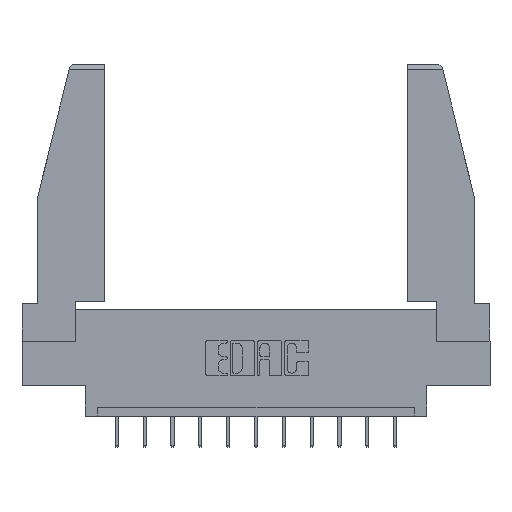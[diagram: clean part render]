
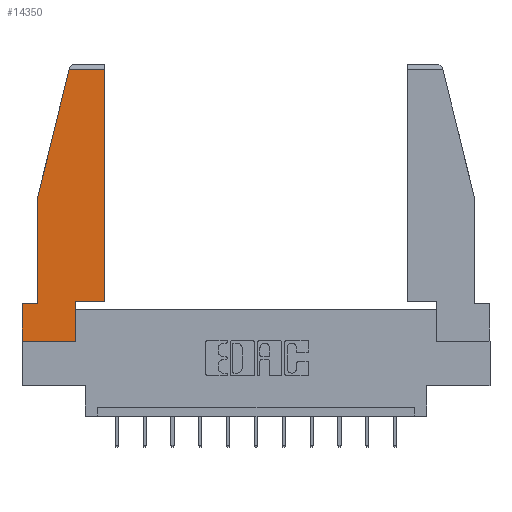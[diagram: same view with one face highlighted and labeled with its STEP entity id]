
A CAD part, top view. The second image highlights one B-rep face of the part: STEP entity #14350.
In plain terms, the highlighted planar face has unit normal (0, 0, 1).
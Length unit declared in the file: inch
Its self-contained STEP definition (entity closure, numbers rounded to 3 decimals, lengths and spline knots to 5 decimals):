
#652 = EDGE_CURVE ( 'NONE', #4869, #4656, #8339, .T. ) ;
#977 = EDGE_CURVE ( 'NONE', #4656, #2754, #12993, .T. ) ;
#1386 = DIRECTION ( 'NONE',  ( 1., 0., 0. ) ) ;
#1557 = ORIENTED_EDGE ( 'NONE', *, *, #977, .T. ) ;
#1839 = VECTOR ( 'NONE', #2332, 39.37008 ) ;
#2135 = FACE_OUTER_BOUND ( 'NONE', #13114, .T. ) ;
#2332 = DIRECTION ( 'NONE',  ( 0., 1., 0. ) ) ;
#2437 = DIRECTION ( 'NONE',  ( -1., 0., 0. ) ) ;
#2501 = DIRECTION ( 'NONE',  ( 0., 1., 0. ) ) ;
#2518 = VERTEX_POINT ( 'NONE', #7886 ) ;
#2739 = ORIENTED_EDGE ( 'NONE', *, *, #652, .T. ) ;
#2754 = VERTEX_POINT ( 'NONE', #12112 ) ;
#3311 = CARTESIAN_POINT ( 'NONE',  ( 0., 0., 0. ) ) ;
#3461 = LINE ( 'NONE', #5971, #7986 ) ;
#3486 = CARTESIAN_POINT ( 'NONE',  ( 0.461, 1.52, 0. ) ) ;
#3615 = DIRECTION ( 'NONE',  ( 0., 0., 1. ) ) ;
#3895 = ORIENTED_EDGE ( 'NONE', *, *, #5594, .T. ) ;
#4079 = ORIENTED_EDGE ( 'NONE', *, *, #12939, .T. ) ;
#4114 = CARTESIAN_POINT ( 'NONE',  ( 0.086, 0.21, 0. ) ) ;
#4650 = VECTOR ( 'NONE', #9243, 39.37008 ) ;
#4656 = VERTEX_POINT ( 'NONE', #4114 ) ;
#4683 = DIRECTION ( 'NONE',  ( 0., -1., 0. ) ) ;
#4845 = VERTEX_POINT ( 'NONE', #10705 ) ;
#4869 = VERTEX_POINT ( 'NONE', #10540 ) ;
#4885 = LINE ( 'NONE', #13971, #1839 ) ;
#4939 = PLANE ( 'NONE',  #11507 ) ;
#5016 = LINE ( 'NONE', #14235, #9665 ) ;
#5052 = CARTESIAN_POINT ( 'NONE',  ( 0.2636, 1.52, 0. ) ) ;
#5412 = ORIENTED_EDGE ( 'NONE', *, *, #7870, .T. ) ;
#5594 = EDGE_CURVE ( 'NONE', #6799, #10793, #7722, .T. ) ;
#5870 = CARTESIAN_POINT ( 'NONE',  ( 0., 0.21, 0. ) ) ;
#5971 = CARTESIAN_POINT ( 'NONE',  ( 0.461, 0.223, 0. ) ) ;
#6303 = ORIENTED_EDGE ( 'NONE', *, *, #13907, .T. ) ;
#6676 = ORIENTED_EDGE ( 'NONE', *, *, #7749, .T. ) ;
#6799 = VERTEX_POINT ( 'NONE', #3311 ) ;
#7091 = CARTESIAN_POINT ( 'NONE',  ( 0., 0., 0. ) ) ;
#7204 = VERTEX_POINT ( 'NONE', #3486 ) ;
#7722 = LINE ( 'NONE', #13910, #4650 ) ;
#7749 = EDGE_CURVE ( 'NONE', #11628, #4869, #10128, .T. ) ;
#7864 = CARTESIAN_POINT ( 'NONE',  ( 0.086, 0.8, 0. ) ) ;
#7870 = EDGE_CURVE ( 'NONE', #4845, #7204, #3461, .T. ) ;
#7886 = CARTESIAN_POINT ( 'NONE',  ( 0.297, 0.223, 0. ) ) ;
#7896 = DIRECTION ( 'NONE',  ( -0.239, -0.971, 0. ) ) ;
#7986 = VECTOR ( 'NONE', #2501, 39.37008 ) ;
#8339 = LINE ( 'NONE', #7864, #13729 ) ;
#8578 = VECTOR ( 'NONE', #13225, 39.37008 ) ;
#8624 = EDGE_CURVE ( 'NONE', #2518, #4845, #12703, .T. ) ;
#9120 = CARTESIAN_POINT ( 'NONE',  ( 0.271, 1.55, 0. ) ) ;
#9243 = DIRECTION ( 'NONE',  ( 1., 0., 0. ) ) ;
#9665 = VECTOR ( 'NONE', #2437, 39.37008 ) ;
#9892 = VECTOR ( 'NONE', #13787, 39.37008 ) ;
#9951 = VECTOR ( 'NONE', #14261, 39.37008 ) ;
#10076 = ORIENTED_EDGE ( 'NONE', *, *, #12726, .T. ) ;
#10128 = LINE ( 'NONE', #9120, #12649 ) ;
#10540 = CARTESIAN_POINT ( 'NONE',  ( 0.086, 0.8, 0. ) ) ;
#10705 = CARTESIAN_POINT ( 'NONE',  ( 0.461, 0.223, 0. ) ) ;
#10793 = VERTEX_POINT ( 'NONE', #13308 ) ;
#11507 = AXIS2_PLACEMENT_3D ( 'NONE', #7091, #3615, #1386 ) ;
#11628 = VERTEX_POINT ( 'NONE', #5052 ) ;
#11841 = ORIENTED_EDGE ( 'NONE', *, *, #8624, .T. ) ;
#12066 = CARTESIAN_POINT ( 'NONE',  ( 0.297, 0.223, 0. ) ) ;
#12112 = CARTESIAN_POINT ( 'NONE',  ( 0., 0.21, 0. ) ) ;
#12594 = LINE ( 'NONE', #5870, #9892 ) ;
#12649 = VECTOR ( 'NONE', #7896, 39.37008 ) ;
#12703 = LINE ( 'NONE', #12066, #8578 ) ;
#12726 = EDGE_CURVE ( 'NONE', #10793, #2518, #4885, .T. ) ;
#12939 = EDGE_CURVE ( 'NONE', #2754, #6799, #12594, .T. ) ;
#12993 = LINE ( 'NONE', #13101, #9951 ) ;
#13101 = CARTESIAN_POINT ( 'NONE',  ( 0., 0.21, 0. ) ) ;
#13114 = EDGE_LOOP ( 'NONE', ( #5412, #6303, #6676, #2739, #1557, #4079, #3895, #10076, #11841 ) ) ;
#13225 = DIRECTION ( 'NONE',  ( 1., 0., 0. ) ) ;
#13308 = CARTESIAN_POINT ( 'NONE',  ( 0.297, 0., 0. ) ) ;
#13729 = VECTOR ( 'NONE', #4683, 39.37008 ) ;
#13787 = DIRECTION ( 'NONE',  ( 0., -1., 0. ) ) ;
#13907 = EDGE_CURVE ( 'NONE', #7204, #11628, #5016, .T. ) ;
#13910 = CARTESIAN_POINT ( 'NONE',  ( 0., 0., 0. ) ) ;
#13971 = CARTESIAN_POINT ( 'NONE',  ( 0.297, 0., 0. ) ) ;
#14235 = CARTESIAN_POINT ( 'NONE',  ( 0., 1.52, 0. ) ) ;
#14261 = DIRECTION ( 'NONE',  ( -1., 0., 0. ) ) ;
#14350 = ADVANCED_FACE ( 'NONE', ( #2135 ), #4939, .T. ) ;
